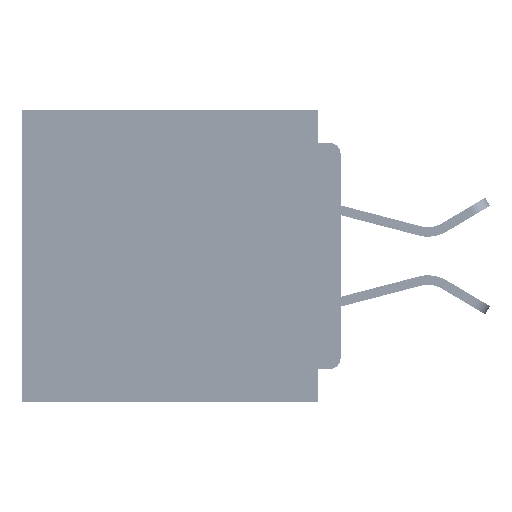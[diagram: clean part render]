
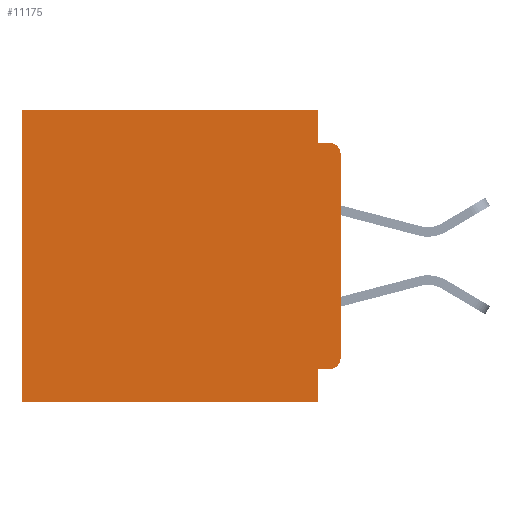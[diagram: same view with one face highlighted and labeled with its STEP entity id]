
A CAD part, left-side view. The second image highlights one B-rep face of the part: STEP entity #11175.
In plain terms, the highlighted planar face has unit normal (-1, 0, 0).
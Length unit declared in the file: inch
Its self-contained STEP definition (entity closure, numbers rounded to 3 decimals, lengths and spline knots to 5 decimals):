
#471 = LINE ( 'NONE', #32201, #51418 ) ;
#832 = CARTESIAN_POINT ( 'NONE',  ( 0.3, 0.015, -0.06 ) ) ;
#1159 = CARTESIAN_POINT ( 'NONE',  ( 0.3, 0., -0.34 ) ) ;
#1185 = CARTESIAN_POINT ( 'NONE',  ( 0.3, 0.031, -0.045 ) ) ;
#1415 = VERTEX_POINT ( 'NONE', #36275 ) ;
#2464 = DIRECTION ( 'NONE',  ( 0., 0., -1. ) ) ;
#2721 = DIRECTION ( 'NONE',  ( 0., 0., -1. ) ) ;
#2931 = VECTOR ( 'NONE', #47199, 39.37008 ) ;
#3255 = VERTEX_POINT ( 'NONE', #13290 ) ;
#3787 = LINE ( 'NONE', #47307, #25278 ) ;
#3872 = VECTOR ( 'NONE', #16737, 39.37008 ) ;
#3946 = CARTESIAN_POINT ( 'NONE',  ( 0.3, 0.031, -0.4 ) ) ;
#4858 = DIRECTION ( 'NONE',  ( 0., 0., -1. ) ) ;
#5644 = EDGE_CURVE ( 'NONE', #25711, #28629, #43672, .T. ) ;
#6793 = CIRCLE ( 'NONE', #41353, 0.015 ) ;
#6974 = LINE ( 'NONE', #45099, #36498 ) ;
#7824 = ORIENTED_EDGE ( 'NONE', *, *, #46624, .F. ) ;
#8462 = CARTESIAN_POINT ( 'NONE',  ( 0.3, 0.031, -0.4 ) ) ;
#9277 = VECTOR ( 'NONE', #10869, 39.37008 ) ;
#10869 = DIRECTION ( 'NONE',  ( 0., -1., 0. ) ) ;
#10874 = DIRECTION ( 'NONE',  ( -1., 0., 0. ) ) ;
#11076 = ORIENTED_EDGE ( 'NONE', *, *, #36728, .T. ) ;
#11175 = ADVANCED_FACE ( 'NONE', ( #50171 ), #30517, .F. ) ;
#13290 = CARTESIAN_POINT ( 'NONE',  ( 0.3, 0.437, 0. ) ) ;
#14520 = CARTESIAN_POINT ( 'NONE',  ( 0.3, 0.437, -0.4 ) ) ;
#15576 = VERTEX_POINT ( 'NONE', #37144 ) ;
#15742 = AXIS2_PLACEMENT_3D ( 'NONE', #34838, #10874, #38916 ) ;
#16009 = DIRECTION ( 'NONE',  ( 0., 0., -1. ) ) ;
#16737 = DIRECTION ( 'NONE',  ( 0., 1., 0. ) ) ;
#16816 = EDGE_CURVE ( 'NONE', #30634, #1415, #6793, .T. ) ;
#17601 = EDGE_CURVE ( 'NONE', #34769, #1415, #19985, .T. ) ;
#17827 = CARTESIAN_POINT ( 'NONE',  ( 0.3, 0., -0.06 ) ) ;
#18801 = ORIENTED_EDGE ( 'NONE', *, *, #16816, .T. ) ;
#19241 = DIRECTION ( 'NONE',  ( 0., 0., -1. ) ) ;
#19985 = LINE ( 'NONE', #26676, #9277 ) ;
#22657 = CARTESIAN_POINT ( 'NONE',  ( 0.3, 0.015, -0.355 ) ) ;
#23634 = VECTOR ( 'NONE', #16009, 39.37008 ) ;
#23996 = VECTOR ( 'NONE', #2464, 39.37008 ) ;
#24408 = LINE ( 'NONE', #47367, #2931 ) ;
#24640 = CARTESIAN_POINT ( 'NONE',  ( 0.3, 0., -0.4 ) ) ;
#25124 = DIRECTION ( 'NONE',  ( 0., 1., 0. ) ) ;
#25278 = VECTOR ( 'NONE', #19241, 39.37008 ) ;
#25711 = VERTEX_POINT ( 'NONE', #40308 ) ;
#26057 = AXIS2_PLACEMENT_3D ( 'NONE', #50895, #26858, #2721 ) ;
#26497 = LINE ( 'NONE', #14520, #23996 ) ;
#26603 = LINE ( 'NONE', #24640, #3872 ) ;
#26676 = CARTESIAN_POINT ( 'NONE',  ( 0.3, 0., -0.045 ) ) ;
#26858 = DIRECTION ( 'NONE',  ( 1., 0., 0. ) ) ;
#28194 = DIRECTION ( 'NONE',  ( 0., 1., 0. ) ) ;
#28629 = VERTEX_POINT ( 'NONE', #8462 ) ;
#29003 = DIRECTION ( 'NONE',  ( -1., 0., 0. ) ) ;
#30517 = PLANE ( 'NONE',  #26057 ) ;
#30634 = VERTEX_POINT ( 'NONE', #17827 ) ;
#30994 = EDGE_CURVE ( 'NONE', #33743, #25711, #471, .T. ) ;
#31422 = ORIENTED_EDGE ( 'NONE', *, *, #48730, .T. ) ;
#31940 = ORIENTED_EDGE ( 'NONE', *, *, #30994, .F. ) ;
#32201 = CARTESIAN_POINT ( 'NONE',  ( 0.3, 0., -0.355 ) ) ;
#33687 = VERTEX_POINT ( 'NONE', #50405 ) ;
#33743 = VERTEX_POINT ( 'NONE', #22657 ) ;
#34769 = VERTEX_POINT ( 'NONE', #1185 ) ;
#34838 = CARTESIAN_POINT ( 'NONE',  ( 0.3, 0.015, -0.34 ) ) ;
#35980 = EDGE_LOOP ( 'NONE', ( #46379, #18801, #38881, #7824, #45689, #11076, #43940, #37987, #31940, #31422 ) ) ;
#36275 = CARTESIAN_POINT ( 'NONE',  ( 0.3, 0.015, -0.045 ) ) ;
#36498 = VECTOR ( 'NONE', #25124, 39.37008 ) ;
#36728 = EDGE_CURVE ( 'NONE', #3255, #33687, #26497, .T. ) ;
#37144 = CARTESIAN_POINT ( 'NONE',  ( 0.3, 0.031, 0. ) ) ;
#37987 = ORIENTED_EDGE ( 'NONE', *, *, #5644, .F. ) ;
#38881 = ORIENTED_EDGE ( 'NONE', *, *, #17601, .F. ) ;
#38916 = DIRECTION ( 'NONE',  ( 0., 0., -1. ) ) ;
#39776 = EDGE_CURVE ( 'NONE', #28629, #33687, #26603, .T. ) ;
#40308 = CARTESIAN_POINT ( 'NONE',  ( 0.3, 0.031, -0.355 ) ) ;
#40389 = EDGE_CURVE ( 'NONE', #15576, #3255, #6974, .T. ) ;
#41313 = EDGE_CURVE ( 'NONE', #30634, #45744, #3787, .T. ) ;
#41353 = AXIS2_PLACEMENT_3D ( 'NONE', #832, #29003, #4858 ) ;
#43672 = LINE ( 'NONE', #3946, #23634 ) ;
#43940 = ORIENTED_EDGE ( 'NONE', *, *, #39776, .F. ) ;
#45099 = CARTESIAN_POINT ( 'NONE',  ( 0.3, 0., 0. ) ) ;
#45689 = ORIENTED_EDGE ( 'NONE', *, *, #40389, .T. ) ;
#45744 = VERTEX_POINT ( 'NONE', #1159 ) ;
#46379 = ORIENTED_EDGE ( 'NONE', *, *, #41313, .F. ) ;
#46624 = EDGE_CURVE ( 'NONE', #15576, #34769, #24408, .T. ) ;
#47199 = DIRECTION ( 'NONE',  ( 0., 0., -1. ) ) ;
#47307 = CARTESIAN_POINT ( 'NONE',  ( 0.3, 0., -0.4 ) ) ;
#47367 = CARTESIAN_POINT ( 'NONE',  ( 0.3, 0.031, 0. ) ) ;
#48721 = CIRCLE ( 'NONE', #15742, 0.015 ) ;
#48730 = EDGE_CURVE ( 'NONE', #33743, #45744, #48721, .T. ) ;
#50171 = FACE_OUTER_BOUND ( 'NONE', #35980, .T. ) ;
#50405 = CARTESIAN_POINT ( 'NONE',  ( 0.3, 0.437, -0.4 ) ) ;
#50895 = CARTESIAN_POINT ( 'NONE',  ( 0.3, 0., -0.4 ) ) ;
#51418 = VECTOR ( 'NONE', #28194, 39.37008 ) ;
